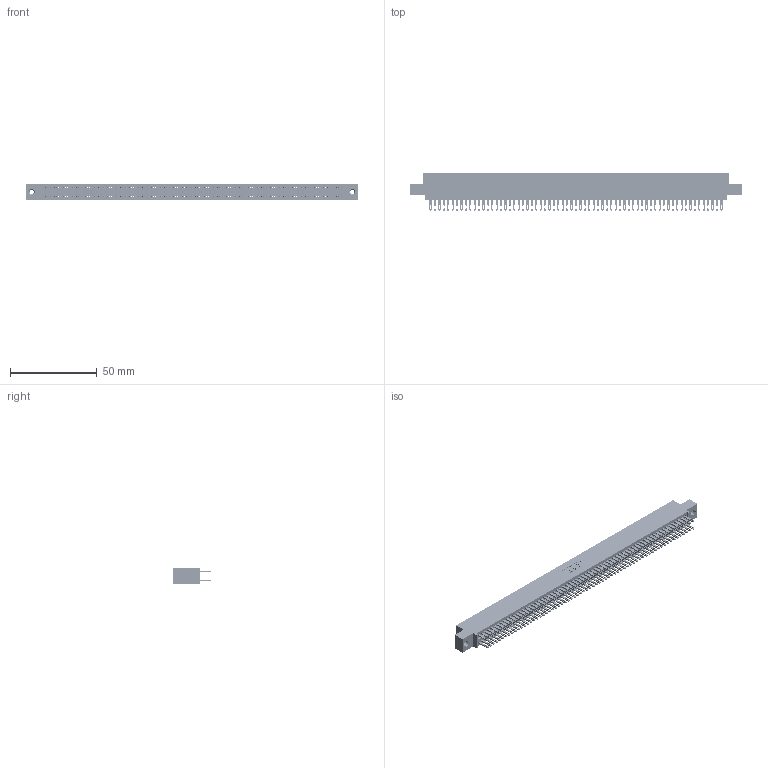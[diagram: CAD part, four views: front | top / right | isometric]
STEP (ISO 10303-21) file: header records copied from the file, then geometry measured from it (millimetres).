
FILE_DESCRIPTION (( 'STEP AP203' ), '1' );
FILE_NAME ('895-134-500-508.STEP', '2020-10-13T18:02:50', ( '' ), ( '' ), 'SwSTEP 2.0', 'SolidWorks 2020', '' );
FILE_SCHEMA (( 'CONFIG_CONTROL_DESIGN' ));
Length unit declared in the file: inch
Products named in the file (4): 345-250-001_345-250-003-102; 845 Part_0.110 Offset - 0.156 Dia-TI; 895-134-500-508; 345-292-001_345-293-100
Assembly tree (137 placements, depth 2):
  895-134-500-508
    845 Part_0.110 Offset - 0.156 Dia-TI
    345-292-001_345-293-100  x134
    345-250-001_345-250-003-102  x2
Bounding box: 191.39 x 21.51 x 9.4 mm (x, y, z)
Volume: 19153.4 mm3; surface area: 30269.1 mm2
Topology: 137 solids, 137 shells, 6354 faces, 19383 edges, 12914 vertices
Faces by surface type: plane 3734, cylinder 2604, cone 12, torus 4
Entity records: 50452 total; most frequent: CARTESIAN_POINT 8415, ORIENTED_EDGE 8342, DIRECTION 7417, EDGE_CURVE 4171, VECTOR 3747, LINE 3747, VERTEX_POINT 2776, AXIS2_PLACEMENT_3D 1835
